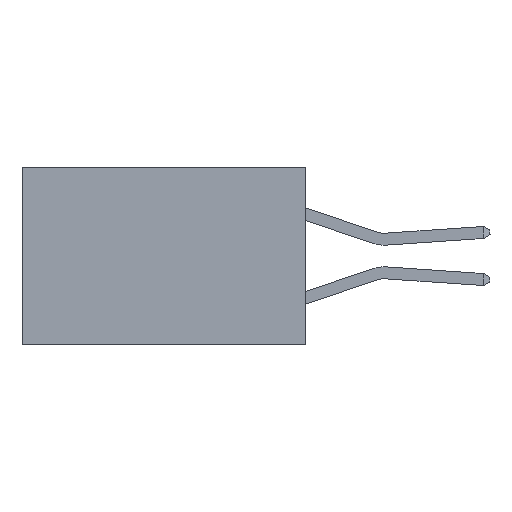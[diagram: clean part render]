
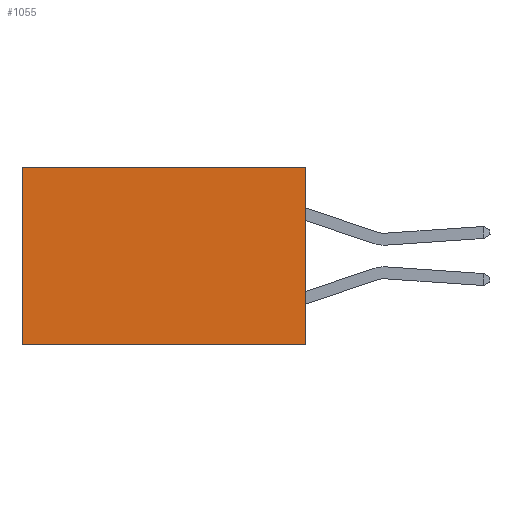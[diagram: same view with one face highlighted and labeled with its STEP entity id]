
A CAD part, left-side view. The second image highlights one B-rep face of the part: STEP entity #1055.
In plain terms, the highlighted planar face has unit normal (-1, 0, 0).
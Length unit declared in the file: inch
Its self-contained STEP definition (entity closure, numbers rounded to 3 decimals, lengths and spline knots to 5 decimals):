
#1055 = ADVANCED_FACE ( 'NONE', ( #9695 ), #8219, .F. ) ;
#2348 = CARTESIAN_POINT ( 'NONE',  ( 0.277, 0., -0.37 ) ) ;
#2739 = VECTOR ( 'NONE', #6083, 39.37008 ) ;
#3263 = DIRECTION ( 'NONE',  ( 0., 0., -1. ) ) ;
#3899 = CARTESIAN_POINT ( 'NONE',  ( 0.277, 0.59, -0.37 ) ) ;
#5272 = LINE ( 'NONE', #10636, #8728 ) ;
#5336 = AXIS2_PLACEMENT_3D ( 'NONE', #2348, #12180, #8600 ) ;
#5540 = EDGE_CURVE ( 'NONE', #14789, #19624, #7003, .T. ) ;
#5577 = DIRECTION ( 'NONE',  ( 0., 1., 0. ) ) ;
#6083 = DIRECTION ( 'NONE',  ( 0., 1., 0. ) ) ;
#6109 = CARTESIAN_POINT ( 'NONE',  ( 0.277, 0., -0.37 ) ) ;
#7003 = LINE ( 'NONE', #6109, #2739 ) ;
#7529 = VERTEX_POINT ( 'NONE', #17127 ) ;
#7758 = LINE ( 'NONE', #11939, #21436 ) ;
#8197 = EDGE_LOOP ( 'NONE', ( #14979, #21657, #9069, #13071 ) ) ;
#8219 = PLANE ( 'NONE',  #5336 ) ;
#8600 = DIRECTION ( 'NONE',  ( 0., 0., -1. ) ) ;
#8728 = VECTOR ( 'NONE', #5577, 39.37008 ) ;
#8952 = EDGE_CURVE ( 'NONE', #7529, #14789, #7758, .T. ) ;
#9069 = ORIENTED_EDGE ( 'NONE', *, *, #8952, .F. ) ;
#9695 = FACE_OUTER_BOUND ( 'NONE', #8197, .T. ) ;
#9935 = EDGE_CURVE ( 'NONE', #20515, #19624, #18548, .T. ) ;
#10636 = CARTESIAN_POINT ( 'NONE',  ( 0.277, 0., 0. ) ) ;
#11353 = EDGE_CURVE ( 'NONE', #7529, #20515, #5272, .T. ) ;
#11939 = CARTESIAN_POINT ( 'NONE',  ( 0.277, 0., -0.37 ) ) ;
#12180 = DIRECTION ( 'NONE',  ( 1., 0., 0. ) ) ;
#12489 = DIRECTION ( 'NONE',  ( 0., 0., -1. ) ) ;
#12494 = CARTESIAN_POINT ( 'NONE',  ( 0.277, 0., -0.37 ) ) ;
#12644 = CARTESIAN_POINT ( 'NONE',  ( 0.277, 0.59, 0. ) ) ;
#13071 = ORIENTED_EDGE ( 'NONE', *, *, #11353, .T. ) ;
#14789 = VERTEX_POINT ( 'NONE', #12494 ) ;
#14979 = ORIENTED_EDGE ( 'NONE', *, *, #9935, .T. ) ;
#16937 = VECTOR ( 'NONE', #12489, 39.37008 ) ;
#17127 = CARTESIAN_POINT ( 'NONE',  ( 0.277, 0., 0. ) ) ;
#17940 = CARTESIAN_POINT ( 'NONE',  ( 0.277, 0.59, -0.37 ) ) ;
#18548 = LINE ( 'NONE', #3899, #16937 ) ;
#19624 = VERTEX_POINT ( 'NONE', #17940 ) ;
#20515 = VERTEX_POINT ( 'NONE', #12644 ) ;
#21436 = VECTOR ( 'NONE', #3263, 39.37008 ) ;
#21657 = ORIENTED_EDGE ( 'NONE', *, *, #5540, .F. ) ;
